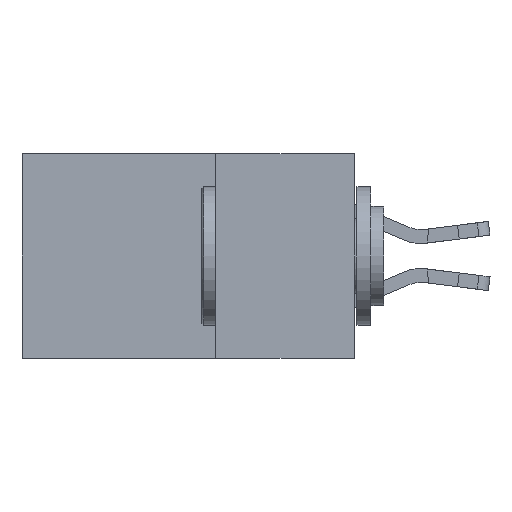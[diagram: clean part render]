
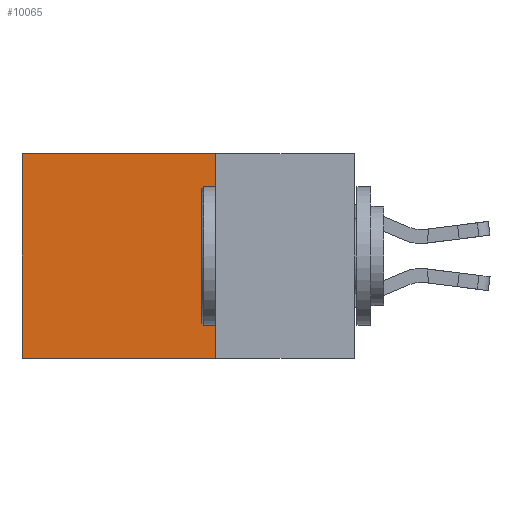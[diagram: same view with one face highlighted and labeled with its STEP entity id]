
A CAD part, left-side view. The second image highlights one B-rep face of the part: STEP entity #10065.
In plain terms, the highlighted planar face has unit normal (-1, 0, 0).
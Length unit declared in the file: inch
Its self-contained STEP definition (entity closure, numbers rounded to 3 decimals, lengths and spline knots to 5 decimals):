
#21 = EDGE_LOOP ( 'NONE', ( #10127, #831, #11350, #6994 ) ) ;
#266 = EDGE_CURVE ( 'NONE', #12718, #3644, #6059, .T. ) ;
#346 = DIRECTION ( 'NONE',  ( 0., 1., 0. ) ) ;
#643 = DIRECTION ( 'NONE',  ( 0., 0., -1. ) ) ;
#762 = VECTOR ( 'NONE', #346, 39.37008 ) ;
#779 = VECTOR ( 'NONE', #1841, 39.37008 ) ;
#831 = ORIENTED_EDGE ( 'NONE', *, *, #11268, .F. ) ;
#1841 = DIRECTION ( 'NONE',  ( 0., 0., -1. ) ) ;
#3389 = CARTESIAN_POINT ( 'NONE',  ( 0.298, 0.6, 0. ) ) ;
#3644 = VERTEX_POINT ( 'NONE', #6594 ) ;
#4621 = DIRECTION ( 'NONE',  ( 1., 0., 0. ) ) ;
#5067 = CARTESIAN_POINT ( 'NONE',  ( 0.298, 0.6, -0.37 ) ) ;
#5633 = CARTESIAN_POINT ( 'NONE',  ( 0.298, 0.25, 0. ) ) ;
#5694 = DIRECTION ( 'NONE',  ( 0., 1., 0. ) ) ;
#5785 = CARTESIAN_POINT ( 'NONE',  ( 0.298, 0.25, 0. ) ) ;
#6051 = LINE ( 'NONE', #11147, #762 ) ;
#6059 = LINE ( 'NONE', #7824, #779 ) ;
#6594 = CARTESIAN_POINT ( 'NONE',  ( 0.298, 0.25, -0.37 ) ) ;
#6994 = ORIENTED_EDGE ( 'NONE', *, *, #8508, .T. ) ;
#7072 = LINE ( 'NONE', #9880, #7845 ) ;
#7548 = CARTESIAN_POINT ( 'NONE',  ( 0.298, 0.6, 0. ) ) ;
#7794 = VECTOR ( 'NONE', #9636, 39.37008 ) ;
#7824 = CARTESIAN_POINT ( 'NONE',  ( 0.298, 0.25, 0. ) ) ;
#7845 = VECTOR ( 'NONE', #5694, 39.37008 ) ;
#8188 = VERTEX_POINT ( 'NONE', #3389 ) ;
#8508 = EDGE_CURVE ( 'NONE', #12718, #8188, #7072, .T. ) ;
#9193 = LINE ( 'NONE', #7548, #7794 ) ;
#9636 = DIRECTION ( 'NONE',  ( 0., 0., -1. ) ) ;
#9880 = CARTESIAN_POINT ( 'NONE',  ( 0.298, 0.25, 0. ) ) ;
#9984 = FACE_OUTER_BOUND ( 'NONE', #21, .T. ) ;
#10010 = EDGE_CURVE ( 'NONE', #8188, #10469, #9193, .T. ) ;
#10065 = ADVANCED_FACE ( 'NONE', ( #9984 ), #12558, .F. ) ;
#10127 = ORIENTED_EDGE ( 'NONE', *, *, #10010, .T. ) ;
#10469 = VERTEX_POINT ( 'NONE', #5067 ) ;
#11147 = CARTESIAN_POINT ( 'NONE',  ( 0.298, 0.25, -0.37 ) ) ;
#11268 = EDGE_CURVE ( 'NONE', #3644, #10469, #6051, .T. ) ;
#11350 = ORIENTED_EDGE ( 'NONE', *, *, #266, .F. ) ;
#11452 = AXIS2_PLACEMENT_3D ( 'NONE', #5633, #4621, #643 ) ;
#12558 = PLANE ( 'NONE',  #11452 ) ;
#12718 = VERTEX_POINT ( 'NONE', #5785 ) ;
